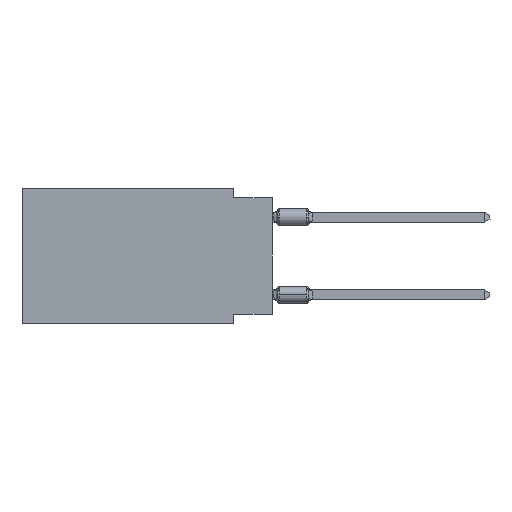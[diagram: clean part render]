
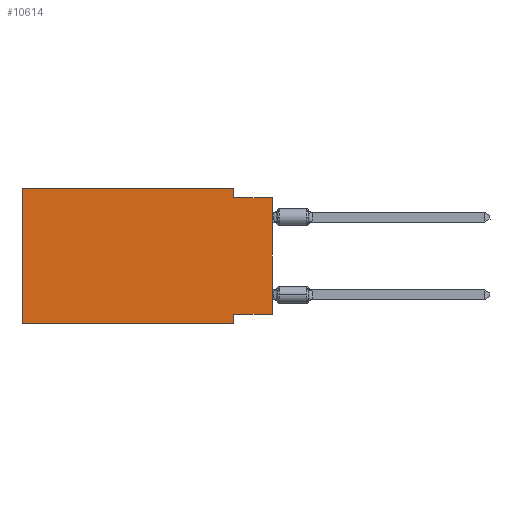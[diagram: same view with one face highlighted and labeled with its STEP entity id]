
A CAD part, left-side view. The second image highlights one B-rep face of the part: STEP entity #10614.
In plain terms, the highlighted planar face has unit normal (-1, 0, 0).
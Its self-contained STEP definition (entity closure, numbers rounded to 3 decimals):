
#355 = EDGE_CURVE ( 'NONE', #12757, #7875, #724, .T. ) ;
#542 = VECTOR ( 'NONE', #1991, 1000. ) ;
#724 = LINE ( 'NONE', #23369, #23371 ) ;
#1070 = CARTESIAN_POINT ( 'NONE',  ( 0., 0., -8.255 ) ) ;
#1991 = DIRECTION ( 'NONE',  ( 0., 0., -1. ) ) ;
#2188 = CARTESIAN_POINT ( 'NONE',  ( 0., 0., -0.635 ) ) ;
#3219 = DIRECTION ( 'NONE',  ( 0., 0., 1. ) ) ;
#3532 = EDGE_LOOP ( 'NONE', ( #9015, #10881, #16306, #22938, #17293, #6750, #19392, #17529 ) ) ;
#3664 = CARTESIAN_POINT ( 'NONE',  ( 0., 0., -8.255 ) ) ;
#4976 = CARTESIAN_POINT ( 'NONE',  ( 0., 16.383, 0. ) ) ;
#5222 = LINE ( 'NONE', #4976, #18945 ) ;
#5296 = DIRECTION ( 'NONE',  ( 1., 0., 0. ) ) ;
#5550 = DIRECTION ( 'NONE',  ( 0., -1., 0. ) ) ;
#5691 = EDGE_CURVE ( 'NONE', #17601, #7906, #6063, .T. ) ;
#6063 = LINE ( 'NONE', #7782, #542 ) ;
#6609 = LINE ( 'NONE', #1070, #9532 ) ;
#6750 = ORIENTED_EDGE ( 'NONE', *, *, #21584, .T. ) ;
#7782 = CARTESIAN_POINT ( 'NONE',  ( 0., 2.54, 0. ) ) ;
#7875 = VERTEX_POINT ( 'NONE', #16555 ) ;
#7906 = VERTEX_POINT ( 'NONE', #21955 ) ;
#8010 = VECTOR ( 'NONE', #9022, 1000. ) ;
#8549 = CARTESIAN_POINT ( 'NONE',  ( 0., 16.383, 0. ) ) ;
#9015 = ORIENTED_EDGE ( 'NONE', *, *, #21477, .T. ) ;
#9022 = DIRECTION ( 'NONE',  ( 0., -1., 0. ) ) ;
#9225 = VECTOR ( 'NONE', #23459, 1000. ) ;
#9532 = VECTOR ( 'NONE', #23235, 1000. ) ;
#10614 = ADVANCED_FACE ( 'NONE', ( #24125 ), #20198, .F. ) ;
#10643 = DIRECTION ( 'NONE',  ( 0., 0., 1. ) ) ;
#10863 = CARTESIAN_POINT ( 'NONE',  ( 0., 0., 0. ) ) ;
#10881 = ORIENTED_EDGE ( 'NONE', *, *, #14178, .F. ) ;
#11484 = VECTOR ( 'NONE', #5550, 1000. ) ;
#11531 = CARTESIAN_POINT ( 'NONE',  ( 0., 2.54, -8.255 ) ) ;
#11998 = VERTEX_POINT ( 'NONE', #14821 ) ;
#12300 = DIRECTION ( 'NONE',  ( 0., 0., -1. ) ) ;
#12757 = VERTEX_POINT ( 'NONE', #11531 ) ;
#12940 = AXIS2_PLACEMENT_3D ( 'NONE', #22162, #5296, #20069 ) ;
#13042 = EDGE_CURVE ( 'NONE', #14079, #17601, #18157, .T. ) ;
#14079 = VERTEX_POINT ( 'NONE', #21965 ) ;
#14178 = EDGE_CURVE ( 'NONE', #7906, #24072, #14233, .T. ) ;
#14233 = LINE ( 'NONE', #15968, #9225 ) ;
#14821 = CARTESIAN_POINT ( 'NONE',  ( 0., 16.383, -8.89 ) ) ;
#15172 = CARTESIAN_POINT ( 'NONE',  ( 0., 16.383, -8.89 ) ) ;
#15411 = VECTOR ( 'NONE', #3219, 1000. ) ;
#15507 = CARTESIAN_POINT ( 'NONE',  ( 0., 2.54, 0. ) ) ;
#15968 = CARTESIAN_POINT ( 'NONE',  ( 0., 0., -0.635 ) ) ;
#16306 = ORIENTED_EDGE ( 'NONE', *, *, #5691, .F. ) ;
#16555 = CARTESIAN_POINT ( 'NONE',  ( 0., 2.54, -8.89 ) ) ;
#17293 = ORIENTED_EDGE ( 'NONE', *, *, #21111, .F. ) ;
#17529 = ORIENTED_EDGE ( 'NONE', *, *, #17641, .F. ) ;
#17601 = VERTEX_POINT ( 'NONE', #15507 ) ;
#17641 = EDGE_CURVE ( 'NONE', #22817, #12757, #6609, .T. ) ;
#18157 = LINE ( 'NONE', #8549, #8010 ) ;
#18945 = VECTOR ( 'NONE', #10643, 1000. ) ;
#19392 = ORIENTED_EDGE ( 'NONE', *, *, #355, .F. ) ;
#20069 = DIRECTION ( 'NONE',  ( 0., 0., -1. ) ) ;
#20198 = PLANE ( 'NONE',  #12940 ) ;
#21111 = EDGE_CURVE ( 'NONE', #11998, #14079, #5222, .T. ) ;
#21477 = EDGE_CURVE ( 'NONE', #22817, #24072, #21812, .T. ) ;
#21584 = EDGE_CURVE ( 'NONE', #11998, #7875, #22416, .T. ) ;
#21812 = LINE ( 'NONE', #10863, #15411 ) ;
#21955 = CARTESIAN_POINT ( 'NONE',  ( 0., 2.54, -0.635 ) ) ;
#21965 = CARTESIAN_POINT ( 'NONE',  ( 0., 16.383, 0. ) ) ;
#22162 = CARTESIAN_POINT ( 'NONE',  ( 0., 16.383, 0. ) ) ;
#22416 = LINE ( 'NONE', #15172, #11484 ) ;
#22817 = VERTEX_POINT ( 'NONE', #3664 ) ;
#22938 = ORIENTED_EDGE ( 'NONE', *, *, #13042, .F. ) ;
#23235 = DIRECTION ( 'NONE',  ( 0., 1., 0. ) ) ;
#23369 = CARTESIAN_POINT ( 'NONE',  ( 0., 2.54, -8.89 ) ) ;
#23371 = VECTOR ( 'NONE', #12300, 1000. ) ;
#23459 = DIRECTION ( 'NONE',  ( 0., -1., 0. ) ) ;
#24072 = VERTEX_POINT ( 'NONE', #2188 ) ;
#24125 = FACE_OUTER_BOUND ( 'NONE', #3532, .T. ) ;
